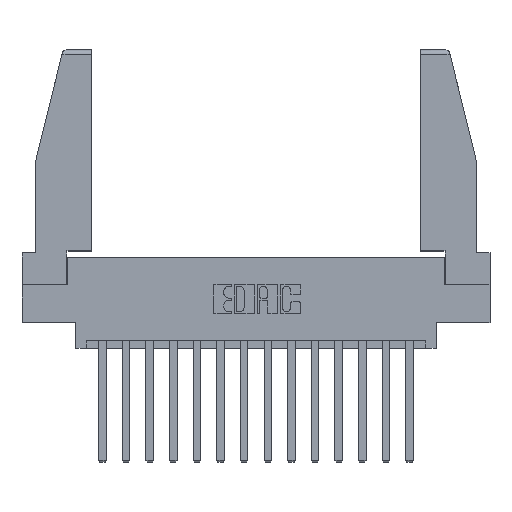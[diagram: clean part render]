
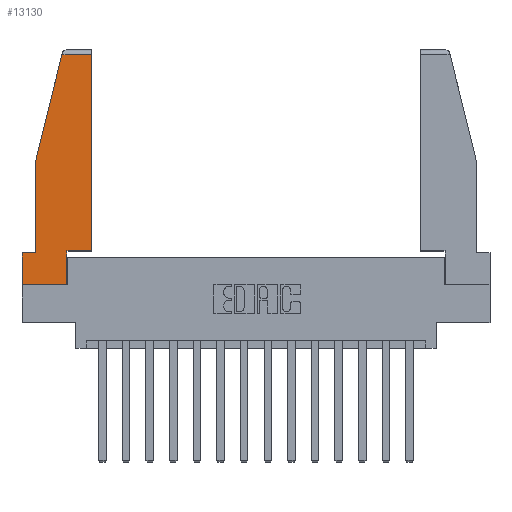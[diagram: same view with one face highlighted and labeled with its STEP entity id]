
A CAD part, top view. The second image highlights one B-rep face of the part: STEP entity #13130.
In plain terms, the highlighted planar face has unit normal (0, 0, 1).
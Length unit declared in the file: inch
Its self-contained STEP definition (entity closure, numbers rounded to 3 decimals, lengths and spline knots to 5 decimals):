
#130 = LINE ( 'NONE', #13281, #13198 ) ;
#337 = CARTESIAN_POINT ( 'NONE',  ( 0., 1.52, 0. ) ) ;
#610 = DIRECTION ( 'NONE',  ( 1., 0., 0. ) ) ;
#622 = CARTESIAN_POINT ( 'NONE',  ( 0.297, 0., 0. ) ) ;
#1444 = LINE ( 'NONE', #12022, #3728 ) ;
#1458 = DIRECTION ( 'NONE',  ( -1., 0., 0. ) ) ;
#1735 = CARTESIAN_POINT ( 'NONE',  ( 0., 0., 0. ) ) ;
#1832 = LINE ( 'NONE', #9476, #12672 ) ;
#2086 = EDGE_LOOP ( 'NONE', ( #5572, #3650, #9096, #14751, #12435, #7517, #15416, #2441, #9425 ) ) ;
#2239 = CARTESIAN_POINT ( 'NONE',  ( 0.086, 0.8, 0. ) ) ;
#2241 = LINE ( 'NONE', #337, #15329 ) ;
#2439 = DIRECTION ( 'NONE',  ( -0.239, -0.971, 0. ) ) ;
#2441 = ORIENTED_EDGE ( 'NONE', *, *, #13429, .T. ) ;
#2737 = VERTEX_POINT ( 'NONE', #622 ) ;
#2789 = DIRECTION ( 'NONE',  ( 0., -1., 0. ) ) ;
#2837 = EDGE_CURVE ( 'NONE', #6358, #14699, #8110, .T. ) ;
#2941 = VERTEX_POINT ( 'NONE', #14247 ) ;
#3034 = EDGE_CURVE ( 'NONE', #11508, #5430, #130, .T. ) ;
#3609 = EDGE_CURVE ( 'NONE', #16153, #7176, #15008, .T. ) ;
#3650 = ORIENTED_EDGE ( 'NONE', *, *, #6920, .T. ) ;
#3728 = VECTOR ( 'NONE', #14633, 39.37008 ) ;
#3770 = CARTESIAN_POINT ( 'NONE',  ( 0.271, 1.55, 0. ) ) ;
#4862 = CARTESIAN_POINT ( 'NONE',  ( 0.461, 1.52, 0. ) ) ;
#5430 = VERTEX_POINT ( 'NONE', #10415 ) ;
#5572 = ORIENTED_EDGE ( 'NONE', *, *, #3609, .T. ) ;
#5735 = DIRECTION ( 'NONE',  ( 0., 0., 1. ) ) ;
#5980 = EDGE_CURVE ( 'NONE', #2941, #16153, #8230, .T. ) ;
#6104 = CARTESIAN_POINT ( 'NONE',  ( 0.461, 0.223, 0. ) ) ;
#6358 = VERTEX_POINT ( 'NONE', #9246 ) ;
#6561 = VERTEX_POINT ( 'NONE', #11611 ) ;
#6913 = CARTESIAN_POINT ( 'NONE',  ( 0., 0., 0. ) ) ;
#6920 = EDGE_CURVE ( 'NONE', #7176, #6358, #2241, .T. ) ;
#6953 = EDGE_CURVE ( 'NONE', #5430, #6561, #1832, .T. ) ;
#7176 = VERTEX_POINT ( 'NONE', #4862 ) ;
#7301 = CARTESIAN_POINT ( 'NONE',  ( 0.086, 0.21, 0. ) ) ;
#7507 = CARTESIAN_POINT ( 'NONE',  ( 0.297, 0.223, 0. ) ) ;
#7517 = ORIENTED_EDGE ( 'NONE', *, *, #6953, .T. ) ;
#7704 = EDGE_CURVE ( 'NONE', #6561, #2737, #10705, .T. ) ;
#7882 = FACE_OUTER_BOUND ( 'NONE', #2086, .T. ) ;
#8110 = LINE ( 'NONE', #3770, #11984 ) ;
#8160 = DIRECTION ( 'NONE',  ( -1., 0., 0. ) ) ;
#8230 = LINE ( 'NONE', #7507, #10472 ) ;
#8449 = PLANE ( 'NONE',  #13032 ) ;
#8673 = VECTOR ( 'NONE', #9587, 39.37008 ) ;
#8825 = DIRECTION ( 'NONE',  ( 1., 0., 0. ) ) ;
#8857 = EDGE_CURVE ( 'NONE', #14699, #11508, #1444, .T. ) ;
#9096 = ORIENTED_EDGE ( 'NONE', *, *, #2837, .T. ) ;
#9142 = LINE ( 'NONE', #12766, #14615 ) ;
#9246 = CARTESIAN_POINT ( 'NONE',  ( 0.2636, 1.52, 0. ) ) ;
#9425 = ORIENTED_EDGE ( 'NONE', *, *, #5980, .T. ) ;
#9476 = CARTESIAN_POINT ( 'NONE',  ( 0., 0.21, 0. ) ) ;
#9587 = DIRECTION ( 'NONE',  ( 1., 0., 0. ) ) ;
#10134 = DIRECTION ( 'NONE',  ( 0., 1., 0. ) ) ;
#10415 = CARTESIAN_POINT ( 'NONE',  ( 0., 0.21, 0. ) ) ;
#10472 = VECTOR ( 'NONE', #8825, 39.37008 ) ;
#10705 = LINE ( 'NONE', #6913, #8673 ) ;
#11508 = VERTEX_POINT ( 'NONE', #7301 ) ;
#11611 = CARTESIAN_POINT ( 'NONE',  ( 0., 0., 0. ) ) ;
#11984 = VECTOR ( 'NONE', #2439, 39.37008 ) ;
#12022 = CARTESIAN_POINT ( 'NONE',  ( 0.086, 0.8, 0. ) ) ;
#12435 = ORIENTED_EDGE ( 'NONE', *, *, #3034, .T. ) ;
#12672 = VECTOR ( 'NONE', #2789, 39.37008 ) ;
#12766 = CARTESIAN_POINT ( 'NONE',  ( 0.297, 0., 0. ) ) ;
#13032 = AXIS2_PLACEMENT_3D ( 'NONE', #1735, #5735, #610 ) ;
#13130 = ADVANCED_FACE ( 'NONE', ( #7882 ), #8449, .T. ) ;
#13167 = CARTESIAN_POINT ( 'NONE',  ( 0.461, 0.223, 0. ) ) ;
#13198 = VECTOR ( 'NONE', #8160, 39.37008 ) ;
#13281 = CARTESIAN_POINT ( 'NONE',  ( 0., 0.21, 0. ) ) ;
#13429 = EDGE_CURVE ( 'NONE', #2737, #2941, #9142, .T. ) ;
#13988 = VECTOR ( 'NONE', #10134, 39.37008 ) ;
#14247 = CARTESIAN_POINT ( 'NONE',  ( 0.297, 0.223, 0. ) ) ;
#14615 = VECTOR ( 'NONE', #16684, 39.37008 ) ;
#14633 = DIRECTION ( 'NONE',  ( 0., -1., 0. ) ) ;
#14699 = VERTEX_POINT ( 'NONE', #2239 ) ;
#14751 = ORIENTED_EDGE ( 'NONE', *, *, #8857, .T. ) ;
#15008 = LINE ( 'NONE', #6104, #13988 ) ;
#15329 = VECTOR ( 'NONE', #1458, 39.37008 ) ;
#15416 = ORIENTED_EDGE ( 'NONE', *, *, #7704, .T. ) ;
#16153 = VERTEX_POINT ( 'NONE', #13167 ) ;
#16684 = DIRECTION ( 'NONE',  ( 0., 1., 0. ) ) ;
